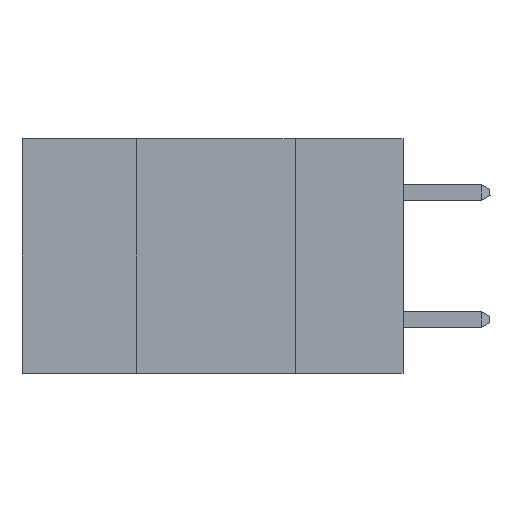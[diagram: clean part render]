
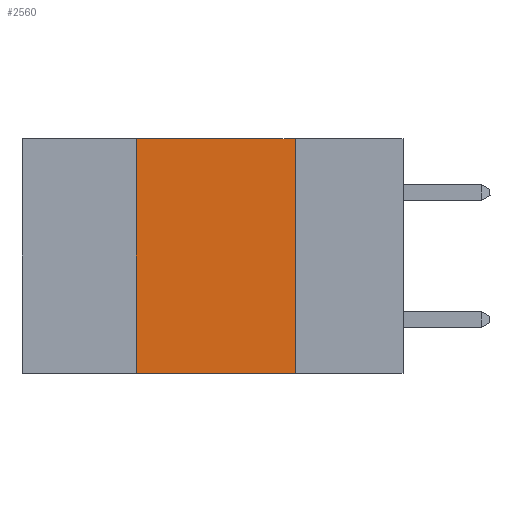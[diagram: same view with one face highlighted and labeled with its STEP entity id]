
A CAD part, left-side view. The second image highlights one B-rep face of the part: STEP entity #2560.
In plain terms, the highlighted planar face has unit normal (-1, 0, 0).
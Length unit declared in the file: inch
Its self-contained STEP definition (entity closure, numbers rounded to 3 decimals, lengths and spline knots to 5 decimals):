
#653 = DIRECTION ( 'NONE',  ( 0., -1., 0. ) ) ;
#756 = CARTESIAN_POINT ( 'NONE',  ( 0., 0.42, 0. ) ) ;
#1934 = ORIENTED_EDGE ( 'NONE', *, *, #17530, .F. ) ;
#2258 = VERTEX_POINT ( 'NONE', #12713 ) ;
#2560 = ADVANCED_FACE ( 'NONE', ( #8114 ), #12341, .F. ) ;
#4334 = LINE ( 'NONE', #10075, #11028 ) ;
#4387 = EDGE_CURVE ( 'NONE', #2258, #16681, #4334, .T. ) ;
#4441 = EDGE_CURVE ( 'NONE', #6783, #16681, #6216, .T. ) ;
#6109 = EDGE_LOOP ( 'NONE', ( #17496, #1934, #9874, #11845 ) ) ;
#6216 = LINE ( 'NONE', #16273, #13756 ) ;
#6509 = DIRECTION ( 'NONE',  ( 1., 0., 0. ) ) ;
#6783 = VERTEX_POINT ( 'NONE', #14916 ) ;
#7532 = EDGE_CURVE ( 'NONE', #6783, #8183, #9805, .T. ) ;
#8114 = FACE_OUTER_BOUND ( 'NONE', #6109, .T. ) ;
#8183 = VERTEX_POINT ( 'NONE', #756 ) ;
#8411 = CARTESIAN_POINT ( 'NONE',  ( 0., 0.42, 0. ) ) ;
#9805 = LINE ( 'NONE', #8411, #10851 ) ;
#9874 = ORIENTED_EDGE ( 'NONE', *, *, #7532, .F. ) ;
#9996 = DIRECTION ( 'NONE',  ( 0., 0., 1. ) ) ;
#10075 = CARTESIAN_POINT ( 'NONE',  ( 0., 0.17, 0. ) ) ;
#10165 = DIRECTION ( 'NONE',  ( 0., 0., -1. ) ) ;
#10851 = VECTOR ( 'NONE', #9996, 39.37008 ) ;
#11028 = VECTOR ( 'NONE', #10165, 39.37008 ) ;
#11700 = CARTESIAN_POINT ( 'NONE',  ( 0., 0.6, 0. ) ) ;
#11845 = ORIENTED_EDGE ( 'NONE', *, *, #4441, .T. ) ;
#12341 = PLANE ( 'NONE',  #15749 ) ;
#12573 = LINE ( 'NONE', #11700, #17923 ) ;
#12710 = CARTESIAN_POINT ( 'NONE',  ( 0., 0.17, -0.37 ) ) ;
#12713 = CARTESIAN_POINT ( 'NONE',  ( 0., 0.17, 0. ) ) ;
#13756 = VECTOR ( 'NONE', #653, 39.37008 ) ;
#14264 = DIRECTION ( 'NONE',  ( 0., -1., 0. ) ) ;
#14916 = CARTESIAN_POINT ( 'NONE',  ( 0., 0.42, -0.37 ) ) ;
#15749 = AXIS2_PLACEMENT_3D ( 'NONE', #17972, #6509, #16739 ) ;
#16273 = CARTESIAN_POINT ( 'NONE',  ( 0., 0.6, -0.37 ) ) ;
#16681 = VERTEX_POINT ( 'NONE', #12710 ) ;
#16739 = DIRECTION ( 'NONE',  ( 0., 0., -1. ) ) ;
#17496 = ORIENTED_EDGE ( 'NONE', *, *, #4387, .F. ) ;
#17530 = EDGE_CURVE ( 'NONE', #8183, #2258, #12573, .T. ) ;
#17923 = VECTOR ( 'NONE', #14264, 39.37008 ) ;
#17972 = CARTESIAN_POINT ( 'NONE',  ( 0., 0.6, 0. ) ) ;
